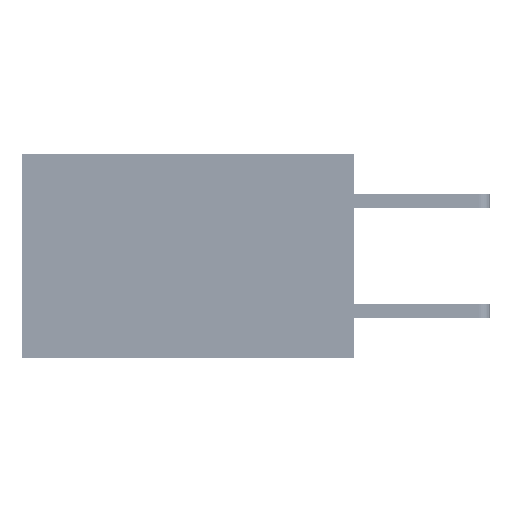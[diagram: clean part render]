
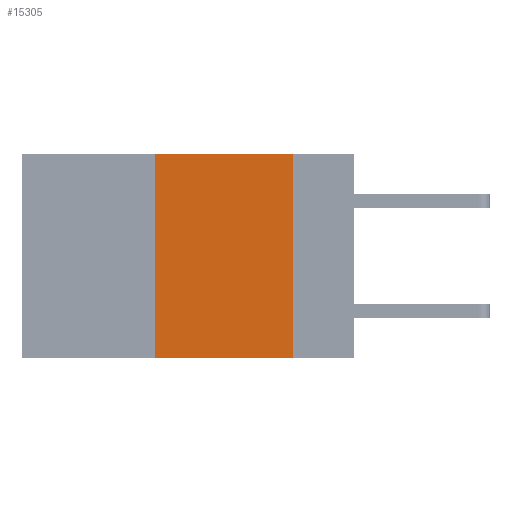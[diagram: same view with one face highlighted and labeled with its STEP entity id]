
A CAD part, left-side view. The second image highlights one B-rep face of the part: STEP entity #15305.
In plain terms, the highlighted planar face has unit normal (-1, 0, 0).
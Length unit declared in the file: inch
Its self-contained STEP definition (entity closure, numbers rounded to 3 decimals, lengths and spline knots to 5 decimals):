
#1064 = DIRECTION ( 'NONE',  ( 0., 0., 1. ) ) ;
#3374 = ORIENTED_EDGE ( 'NONE', *, *, #14188, .T. ) ;
#3955 = DIRECTION ( 'NONE',  ( 0., 0., -1. ) ) ;
#4717 = LINE ( 'NONE', #10830, #25105 ) ;
#5366 = VERTEX_POINT ( 'NONE', #6450 ) ;
#5992 = LINE ( 'NONE', #38077, #10354 ) ;
#6450 = CARTESIAN_POINT ( 'NONE',  ( 0., 0.36, 0. ) ) ;
#8053 = LINE ( 'NONE', #32040, #40067 ) ;
#8322 = EDGE_CURVE ( 'NONE', #35279, #11596, #8053, .T. ) ;
#9420 = EDGE_LOOP ( 'NONE', ( #26346, #25085, #30298, #3374 ) ) ;
#10165 = DIRECTION ( 'NONE',  ( 0., -1., 0. ) ) ;
#10354 = VECTOR ( 'NONE', #10165, 39.37008 ) ;
#10830 = CARTESIAN_POINT ( 'NONE',  ( 0., 0.6, -0.37 ) ) ;
#11596 = VERTEX_POINT ( 'NONE', #19687 ) ;
#13048 = CARTESIAN_POINT ( 'NONE',  ( 0., 0.6, 0. ) ) ;
#13699 = LINE ( 'NONE', #29018, #18042 ) ;
#13788 = CARTESIAN_POINT ( 'NONE',  ( 0., 0.11, 0. ) ) ;
#13951 = DIRECTION ( 'NONE',  ( 0., -1., 0. ) ) ;
#14188 = EDGE_CURVE ( 'NONE', #17113, #11596, #4717, .T. ) ;
#15305 = ADVANCED_FACE ( 'NONE', ( #28000 ), #25112, .F. ) ;
#16289 = AXIS2_PLACEMENT_3D ( 'NONE', #13048, #25501, #22392 ) ;
#17113 = VERTEX_POINT ( 'NONE', #26048 ) ;
#18042 = VECTOR ( 'NONE', #1064, 39.37008 ) ;
#19687 = CARTESIAN_POINT ( 'NONE',  ( 0., 0.11, -0.37 ) ) ;
#22392 = DIRECTION ( 'NONE',  ( 0., 0., -1. ) ) ;
#25085 = ORIENTED_EDGE ( 'NONE', *, *, #33215, .F. ) ;
#25105 = VECTOR ( 'NONE', #13951, 39.37008 ) ;
#25112 = PLANE ( 'NONE',  #16289 ) ;
#25501 = DIRECTION ( 'NONE',  ( 1., 0., 0. ) ) ;
#26048 = CARTESIAN_POINT ( 'NONE',  ( 0., 0.36, -0.37 ) ) ;
#26346 = ORIENTED_EDGE ( 'NONE', *, *, #8322, .F. ) ;
#28000 = FACE_OUTER_BOUND ( 'NONE', #9420, .T. ) ;
#29018 = CARTESIAN_POINT ( 'NONE',  ( 0., 0.36, 0. ) ) ;
#30298 = ORIENTED_EDGE ( 'NONE', *, *, #39761, .F. ) ;
#32040 = CARTESIAN_POINT ( 'NONE',  ( 0., 0.11, 0. ) ) ;
#33215 = EDGE_CURVE ( 'NONE', #5366, #35279, #5992, .T. ) ;
#35279 = VERTEX_POINT ( 'NONE', #13788 ) ;
#38077 = CARTESIAN_POINT ( 'NONE',  ( 0., 0.6, 0. ) ) ;
#39761 = EDGE_CURVE ( 'NONE', #17113, #5366, #13699, .T. ) ;
#40067 = VECTOR ( 'NONE', #3955, 39.37008 ) ;
